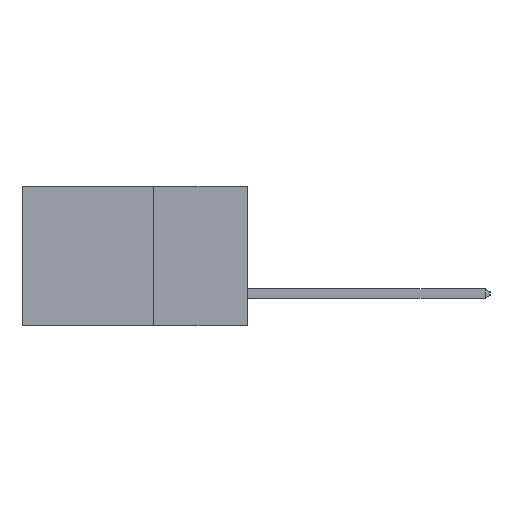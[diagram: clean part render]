
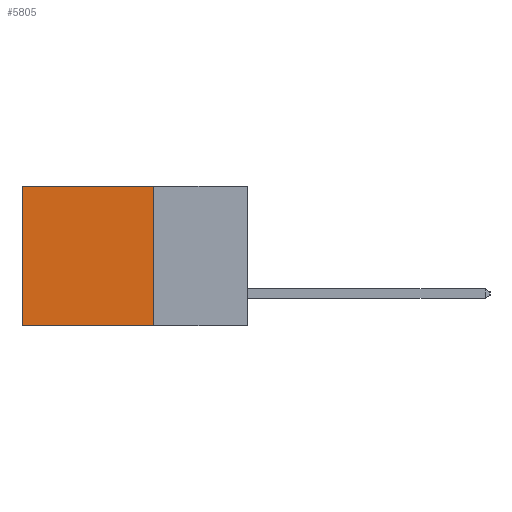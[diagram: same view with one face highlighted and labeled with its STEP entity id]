
A CAD part, left-side view. The second image highlights one B-rep face of the part: STEP entity #5805.
In plain terms, the highlighted planar face has unit normal (-1, 0, 0).
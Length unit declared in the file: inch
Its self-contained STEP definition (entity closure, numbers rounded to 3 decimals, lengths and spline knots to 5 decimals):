
#188 = VERTEX_POINT ( 'NONE', #6629 ) ;
#364 = LINE ( 'NONE', #1192, #3404 ) ;
#1021 = DIRECTION ( 'NONE',  ( 1., 0., 0. ) ) ;
#1192 = CARTESIAN_POINT ( 'NONE',  ( 0.298, 0.25, -0.37 ) ) ;
#1465 = EDGE_CURVE ( 'NONE', #11166, #6767, #16519, .T. ) ;
#1680 = CARTESIAN_POINT ( 'NONE',  ( 0.298, 0.25, 0. ) ) ;
#2321 = FACE_OUTER_BOUND ( 'NONE', #16575, .T. ) ;
#2403 = EDGE_CURVE ( 'NONE', #7623, #188, #364, .T. ) ;
#2421 = VECTOR ( 'NONE', #16393, 39.37008 ) ;
#3404 = VECTOR ( 'NONE', #18157, 39.37008 ) ;
#5763 = VECTOR ( 'NONE', #8733, 39.37008 ) ;
#5805 = ADVANCED_FACE ( 'NONE', ( #2321 ), #17128, .F. ) ;
#6536 = ORIENTED_EDGE ( 'NONE', *, *, #9629, .T. ) ;
#6629 = CARTESIAN_POINT ( 'NONE',  ( 0.298, 0.6, -0.37 ) ) ;
#6767 = VERTEX_POINT ( 'NONE', #13868 ) ;
#7569 = ORIENTED_EDGE ( 'NONE', *, *, #2403, .F. ) ;
#7623 = VERTEX_POINT ( 'NONE', #16027 ) ;
#7669 = CARTESIAN_POINT ( 'NONE',  ( 0.298, 0.25, 0. ) ) ;
#8733 = DIRECTION ( 'NONE',  ( 0., 0., -1. ) ) ;
#9629 = EDGE_CURVE ( 'NONE', #6767, #188, #13589, .T. ) ;
#9911 = CARTESIAN_POINT ( 'NONE',  ( 0.298, 0.25, 0. ) ) ;
#10510 = CARTESIAN_POINT ( 'NONE',  ( 0.298, 0.25, 0. ) ) ;
#11166 = VERTEX_POINT ( 'NONE', #7669 ) ;
#11395 = DIRECTION ( 'NONE',  ( 0., 0., -1. ) ) ;
#12159 = AXIS2_PLACEMENT_3D ( 'NONE', #9911, #1021, #11395 ) ;
#13589 = LINE ( 'NONE', #16040, #5763 ) ;
#13868 = CARTESIAN_POINT ( 'NONE',  ( 0.298, 0.6, 0. ) ) ;
#14215 = LINE ( 'NONE', #1680, #2421 ) ;
#14224 = ORIENTED_EDGE ( 'NONE', *, *, #1465, .T. ) ;
#15479 = ORIENTED_EDGE ( 'NONE', *, *, #16646, .F. ) ;
#16027 = CARTESIAN_POINT ( 'NONE',  ( 0.298, 0.25, -0.37 ) ) ;
#16040 = CARTESIAN_POINT ( 'NONE',  ( 0.298, 0.6, 0. ) ) ;
#16087 = VECTOR ( 'NONE', #17885, 39.37008 ) ;
#16393 = DIRECTION ( 'NONE',  ( 0., 0., -1. ) ) ;
#16519 = LINE ( 'NONE', #10510, #16087 ) ;
#16575 = EDGE_LOOP ( 'NONE', ( #6536, #7569, #15479, #14224 ) ) ;
#16646 = EDGE_CURVE ( 'NONE', #11166, #7623, #14215, .T. ) ;
#17128 = PLANE ( 'NONE',  #12159 ) ;
#17885 = DIRECTION ( 'NONE',  ( 0., 1., 0. ) ) ;
#18157 = DIRECTION ( 'NONE',  ( 0., 1., 0. ) ) ;
